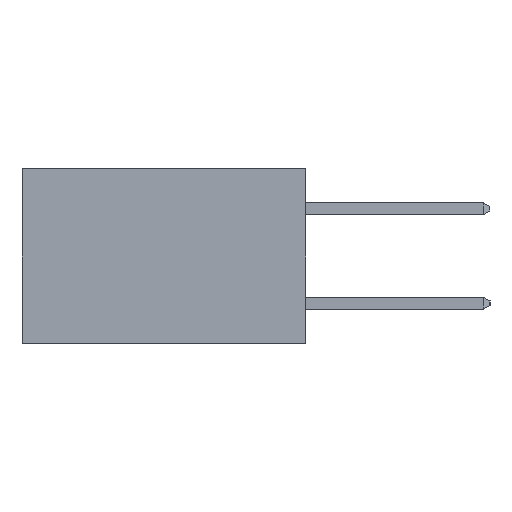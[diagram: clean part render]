
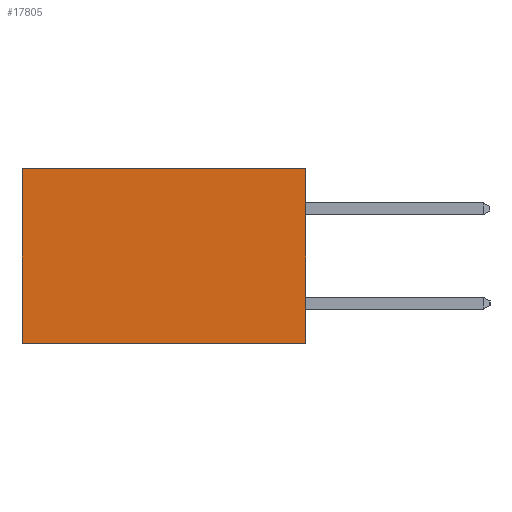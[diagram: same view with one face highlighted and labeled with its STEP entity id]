
A CAD part, left-side view. The second image highlights one B-rep face of the part: STEP entity #17805.
In plain terms, the highlighted planar face has unit normal (-1, 0, 0).
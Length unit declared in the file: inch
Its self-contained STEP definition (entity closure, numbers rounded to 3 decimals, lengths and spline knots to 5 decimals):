
#904 = DIRECTION ( 'NONE',  ( 0., 1., 0. ) ) ;
#1676 = VERTEX_POINT ( 'NONE', #7444 ) ;
#1932 = EDGE_CURVE ( 'NONE', #1676, #8512, #2968, .T. ) ;
#2676 = PLANE ( 'NONE',  #16934 ) ;
#2968 = LINE ( 'NONE', #12592, #10292 ) ;
#3185 = ORIENTED_EDGE ( 'NONE', *, *, #1932, .T. ) ;
#3274 = VECTOR ( 'NONE', #7754, 39.37008 ) ;
#3319 = CARTESIAN_POINT ( 'NONE',  ( 0.2615, 0., -0.37 ) ) ;
#3327 = EDGE_CURVE ( 'NONE', #4309, #1676, #16674, .T. ) ;
#3751 = LINE ( 'NONE', #3319, #3274 ) ;
#4214 = DIRECTION ( 'NONE',  ( 0., 0., -1. ) ) ;
#4309 = VERTEX_POINT ( 'NONE', #17765 ) ;
#5532 = VERTEX_POINT ( 'NONE', #7198 ) ;
#6178 = CARTESIAN_POINT ( 'NONE',  ( 0.2615, 0., -0.37 ) ) ;
#7198 = CARTESIAN_POINT ( 'NONE',  ( 0.2615, 0., -0.37 ) ) ;
#7444 = CARTESIAN_POINT ( 'NONE',  ( 0.2615, 0.6, 0. ) ) ;
#7754 = DIRECTION ( 'NONE',  ( 0., 0., -1. ) ) ;
#8512 = VERTEX_POINT ( 'NONE', #10312 ) ;
#9237 = ORIENTED_EDGE ( 'NONE', *, *, #3327, .T. ) ;
#9357 = EDGE_CURVE ( 'NONE', #4309, #5532, #3751, .T. ) ;
#9801 = VECTOR ( 'NONE', #904, 39.37008 ) ;
#10292 = VECTOR ( 'NONE', #11588, 39.37008 ) ;
#10312 = CARTESIAN_POINT ( 'NONE',  ( 0.2615, 0.6, -0.37 ) ) ;
#10382 = LINE ( 'NONE', #6178, #10828 ) ;
#10828 = VECTOR ( 'NONE', #14555, 39.37008 ) ;
#11349 = CARTESIAN_POINT ( 'NONE',  ( 0.2615, 0., -0.37 ) ) ;
#11588 = DIRECTION ( 'NONE',  ( 0., 0., -1. ) ) ;
#12592 = CARTESIAN_POINT ( 'NONE',  ( 0.2615, 0.6, -0.37 ) ) ;
#12674 = FACE_OUTER_BOUND ( 'NONE', #18506, .T. ) ;
#12796 = DIRECTION ( 'NONE',  ( 1., 0., 0. ) ) ;
#14555 = DIRECTION ( 'NONE',  ( 0., 1., 0. ) ) ;
#14691 = ORIENTED_EDGE ( 'NONE', *, *, #9357, .F. ) ;
#14924 = EDGE_CURVE ( 'NONE', #5532, #8512, #10382, .T. ) ;
#16025 = ORIENTED_EDGE ( 'NONE', *, *, #14924, .F. ) ;
#16674 = LINE ( 'NONE', #17350, #9801 ) ;
#16934 = AXIS2_PLACEMENT_3D ( 'NONE', #11349, #12796, #4214 ) ;
#17350 = CARTESIAN_POINT ( 'NONE',  ( 0.2615, 0., 0. ) ) ;
#17765 = CARTESIAN_POINT ( 'NONE',  ( 0.2615, 0., 0. ) ) ;
#17805 = ADVANCED_FACE ( 'NONE', ( #12674 ), #2676, .F. ) ;
#18506 = EDGE_LOOP ( 'NONE', ( #3185, #16025, #14691, #9237 ) ) ;
